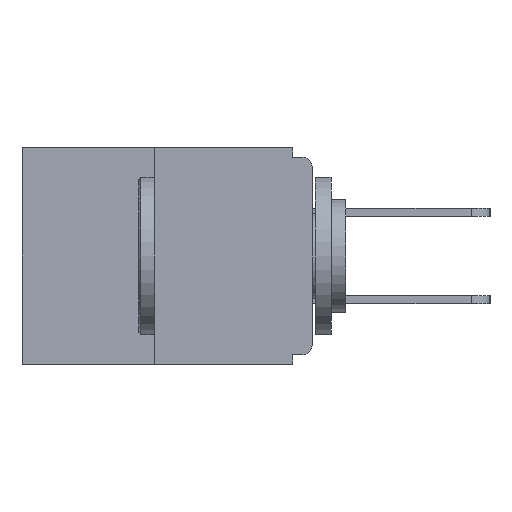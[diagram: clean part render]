
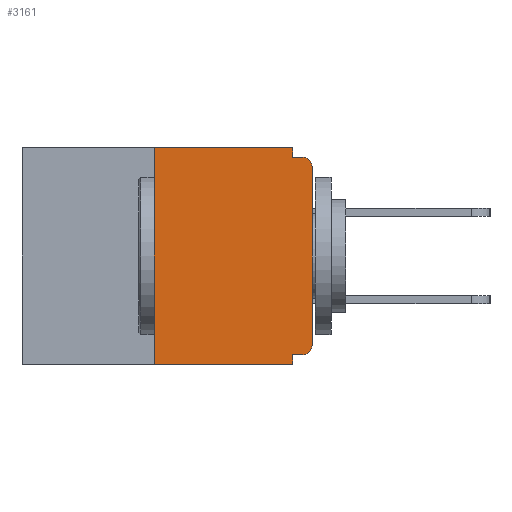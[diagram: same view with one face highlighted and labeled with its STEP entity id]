
A CAD part, left-side view. The second image highlights one B-rep face of the part: STEP entity #3161.
In plain terms, the highlighted planar face has unit normal (-1, 0, 0).
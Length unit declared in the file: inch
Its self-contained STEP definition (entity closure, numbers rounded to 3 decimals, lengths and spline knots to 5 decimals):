
#148 = EDGE_CURVE ( 'NONE', #21871, #11578, #12496, .T. ) ;
#193 = CARTESIAN_POINT ( 'NONE',  ( 0., 0.015, -0.03 ) ) ;
#464 = ORIENTED_EDGE ( 'NONE', *, *, #7261, .F. ) ;
#630 = ORIENTED_EDGE ( 'NONE', *, *, #11050, .F. ) ;
#781 = DIRECTION ( 'NONE',  ( 0., -1., 0. ) ) ;
#888 = DIRECTION ( 'NONE',  ( 0., 0., -1. ) ) ;
#1461 = LINE ( 'NONE', #26439, #3434 ) ;
#1546 = DIRECTION ( 'NONE',  ( -1., 0., 0. ) ) ;
#1606 = ORIENTED_EDGE ( 'NONE', *, *, #6238, .T. ) ;
#1732 = DIRECTION ( 'NONE',  ( 0., 0., -1. ) ) ;
#1834 = CARTESIAN_POINT ( 'NONE',  ( 0., 0.46, -0.343 ) ) ;
#1982 = EDGE_LOOP ( 'NONE', ( #630, #20732, #27034, #25873, #8946, #8803, #1606, #5231, #464, #3445 ) ) ;
#3161 = ADVANCED_FACE ( 'NONE', ( #16290 ), #9420, .F. ) ;
#3383 = CARTESIAN_POINT ( 'NONE',  ( 0., 0.46, 0. ) ) ;
#3434 = VECTOR ( 'NONE', #888, 39.37008 ) ;
#3445 = ORIENTED_EDGE ( 'NONE', *, *, #8034, .F. ) ;
#3776 = VECTOR ( 'NONE', #13595, 39.37008 ) ;
#5231 = ORIENTED_EDGE ( 'NONE', *, *, #148, .T. ) ;
#5393 = DIRECTION ( 'NONE',  ( 0., 0., -1. ) ) ;
#5750 = CARTESIAN_POINT ( 'NONE',  ( 0., 0.031, -0.343 ) ) ;
#6238 = EDGE_CURVE ( 'NONE', #24191, #21871, #26297, .T. ) ;
#6327 = DIRECTION ( 'NONE',  ( 0., 0., 1. ) ) ;
#6890 = VERTEX_POINT ( 'NONE', #12006 ) ;
#7187 = CIRCLE ( 'NONE', #11516, 0.015 ) ;
#7261 = EDGE_CURVE ( 'NONE', #13696, #11578, #20617, .T. ) ;
#7577 = DIRECTION ( 'NONE',  ( 0., 0., -1. ) ) ;
#7741 = VECTOR ( 'NONE', #10752, 39.37008 ) ;
#8034 = EDGE_CURVE ( 'NONE', #8971, #13696, #1461, .T. ) ;
#8038 = EDGE_CURVE ( 'NONE', #17188, #14084, #20597, .T. ) ;
#8653 = DIRECTION ( 'NONE',  ( 0., 0., -1. ) ) ;
#8803 = ORIENTED_EDGE ( 'NONE', *, *, #14955, .T. ) ;
#8946 = ORIENTED_EDGE ( 'NONE', *, *, #8038, .F. ) ;
#8971 = VERTEX_POINT ( 'NONE', #10689 ) ;
#9420 = PLANE ( 'NONE',  #15209 ) ;
#9630 = VERTEX_POINT ( 'NONE', #17761 ) ;
#10384 = CARTESIAN_POINT ( 'NONE',  ( 0., 0., 0. ) ) ;
#10689 = CARTESIAN_POINT ( 'NONE',  ( 0., 0.031, 0. ) ) ;
#10750 = LINE ( 'NONE', #1834, #23298 ) ;
#10752 = DIRECTION ( 'NONE',  ( 0., 0., 1. ) ) ;
#10866 = CARTESIAN_POINT ( 'NONE',  ( 0., 0.25, -0.343 ) ) ;
#11050 = EDGE_CURVE ( 'NONE', #9630, #8971, #23520, .T. ) ;
#11436 = AXIS2_PLACEMENT_3D ( 'NONE', #193, #23856, #8653 ) ;
#11516 = AXIS2_PLACEMENT_3D ( 'NONE', #18270, #1546, #1732 ) ;
#11578 = VERTEX_POINT ( 'NONE', #17215 ) ;
#11789 = EDGE_CURVE ( 'NONE', #14084, #6890, #17292, .T. ) ;
#12006 = CARTESIAN_POINT ( 'NONE',  ( 0., 0.031, -0.343 ) ) ;
#12164 = DIRECTION ( 'NONE',  ( 0., -1., 0. ) ) ;
#12408 = DIRECTION ( 'NONE',  ( 0., -1., 0. ) ) ;
#12496 = CIRCLE ( 'NONE', #11436, 0.015 ) ;
#12844 = LINE ( 'NONE', #23050, #17091 ) ;
#13595 = DIRECTION ( 'NONE',  ( 0., 1., 0. ) ) ;
#13696 = VERTEX_POINT ( 'NONE', #19893 ) ;
#14084 = VERTEX_POINT ( 'NONE', #15162 ) ;
#14955 = EDGE_CURVE ( 'NONE', #17188, #24191, #7187, .T. ) ;
#15162 = CARTESIAN_POINT ( 'NONE',  ( 0., 0.031, -0.328 ) ) ;
#15209 = AXIS2_PLACEMENT_3D ( 'NONE', #3383, #18009, #5393 ) ;
#15691 = CARTESIAN_POINT ( 'NONE',  ( 0., 0.46, 0. ) ) ;
#16290 = FACE_OUTER_BOUND ( 'NONE', #1982, .T. ) ;
#16851 = VECTOR ( 'NONE', #781, 39.37008 ) ;
#16971 = VECTOR ( 'NONE', #7577, 39.37008 ) ;
#17091 = VECTOR ( 'NONE', #6327, 39.37008 ) ;
#17188 = VERTEX_POINT ( 'NONE', #18711 ) ;
#17215 = CARTESIAN_POINT ( 'NONE',  ( 0., 0.015, -0.015 ) ) ;
#17292 = LINE ( 'NONE', #5750, #16971 ) ;
#17761 = CARTESIAN_POINT ( 'NONE',  ( 0., 0.25, 0. ) ) ;
#17876 = CARTESIAN_POINT ( 'NONE',  ( 0., 0., -0.328 ) ) ;
#18009 = DIRECTION ( 'NONE',  ( 1., 0., 0. ) ) ;
#18270 = CARTESIAN_POINT ( 'NONE',  ( 0., 0.015, -0.313 ) ) ;
#18711 = CARTESIAN_POINT ( 'NONE',  ( 0., 0.015, -0.328 ) ) ;
#18770 = CARTESIAN_POINT ( 'NONE',  ( 0., 0., -0.313 ) ) ;
#19290 = VECTOR ( 'NONE', #12164, 39.37008 ) ;
#19893 = CARTESIAN_POINT ( 'NONE',  ( 0., 0.031, -0.015 ) ) ;
#20597 = LINE ( 'NONE', #17876, #3776 ) ;
#20617 = LINE ( 'NONE', #20733, #19290 ) ;
#20732 = ORIENTED_EDGE ( 'NONE', *, *, #21244, .F. ) ;
#20733 = CARTESIAN_POINT ( 'NONE',  ( 0., 0., -0.015 ) ) ;
#21244 = EDGE_CURVE ( 'NONE', #22184, #9630, #12844, .T. ) ;
#21871 = VERTEX_POINT ( 'NONE', #23280 ) ;
#22184 = VERTEX_POINT ( 'NONE', #10866 ) ;
#23050 = CARTESIAN_POINT ( 'NONE',  ( 0., 0.25, 0. ) ) ;
#23280 = CARTESIAN_POINT ( 'NONE',  ( 0., 0., -0.03 ) ) ;
#23298 = VECTOR ( 'NONE', #12408, 39.37008 ) ;
#23520 = LINE ( 'NONE', #15691, #16851 ) ;
#23856 = DIRECTION ( 'NONE',  ( -1., 0., 0. ) ) ;
#24191 = VERTEX_POINT ( 'NONE', #18770 ) ;
#25079 = EDGE_CURVE ( 'NONE', #22184, #6890, #10750, .T. ) ;
#25873 = ORIENTED_EDGE ( 'NONE', *, *, #11789, .F. ) ;
#26297 = LINE ( 'NONE', #10384, #7741 ) ;
#26439 = CARTESIAN_POINT ( 'NONE',  ( 0., 0.031, 0. ) ) ;
#27034 = ORIENTED_EDGE ( 'NONE', *, *, #25079, .T. ) ;
